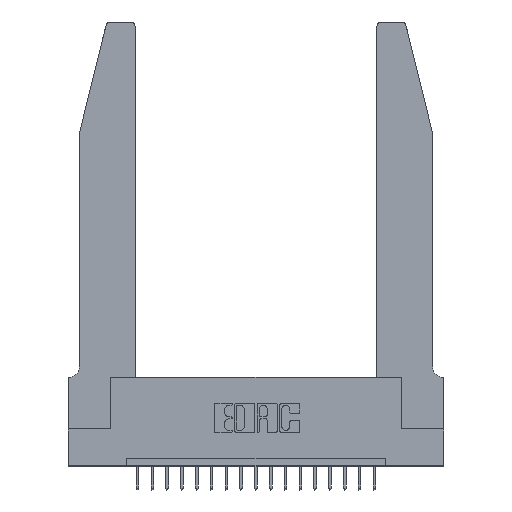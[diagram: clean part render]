
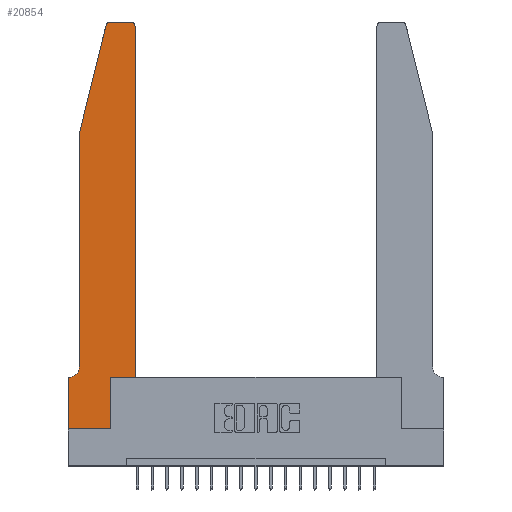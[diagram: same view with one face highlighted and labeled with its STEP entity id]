
A CAD part, top view. The second image highlights one B-rep face of the part: STEP entity #20854.
In plain terms, the highlighted planar face has unit normal (0, 0, 1).
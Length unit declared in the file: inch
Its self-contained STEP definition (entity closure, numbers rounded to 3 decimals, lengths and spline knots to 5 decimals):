
#15 = LINE ( 'NONE', #16925, #7420 ) ;
#464 = DIRECTION ( 'NONE',  ( 0., -1., 0. ) ) ;
#474 = AXIS2_PLACEMENT_3D ( 'NONE', #9435, #6072, #2661 ) ;
#480 = CARTESIAN_POINT ( 'NONE',  ( 0.2865, 0., 0.37 ) ) ;
#1028 = EDGE_CURVE ( 'NONE', #16431, #11741, #10587, .T. ) ;
#1708 = ORIENTED_EDGE ( 'NONE', *, *, #16423, .T. ) ;
#1727 = VERTEX_POINT ( 'NONE', #14026 ) ;
#1805 = CARTESIAN_POINT ( 'NONE',  ( 0.0055, 0.42, 0.37 ) ) ;
#1890 = CARTESIAN_POINT ( 'NONE',  ( 0., 0., 0.37 ) ) ;
#2116 = DIRECTION ( 'NONE',  ( 1., 0., 0. ) ) ;
#2201 = VERTEX_POINT ( 'NONE', #8474 ) ;
#2258 = CARTESIAN_POINT ( 'NONE',  ( 0., 0., 0.37 ) ) ;
#2293 = EDGE_CURVE ( 'NONE', #2201, #3261, #15, .T. ) ;
#2320 = VECTOR ( 'NONE', #464, 39.37008 ) ;
#2518 = FACE_OUTER_BOUND ( 'NONE', #15224, .T. ) ;
#2556 = CARTESIAN_POINT ( 'NONE',  ( 0., 0.35, 0.37 ) ) ;
#2661 = DIRECTION ( 'NONE',  ( 1., 0., 0. ) ) ;
#3010 = EDGE_CURVE ( 'NONE', #5892, #1727, #13741, .T. ) ;
#3032 = LINE ( 'NONE', #14347, #5075 ) ;
#3044 = LINE ( 'NONE', #14842, #20291 ) ;
#3221 = VECTOR ( 'NONE', #3913, 39.37008 ) ;
#3261 = VERTEX_POINT ( 'NONE', #12353 ) ;
#3759 = EDGE_CURVE ( 'NONE', #8178, #20922, #3044, .T. ) ;
#3877 = DIRECTION ( 'NONE',  ( 0., 0., 1. ) ) ;
#3913 = DIRECTION ( 'NONE',  ( -1., 0., 0. ) ) ;
#4110 = ORIENTED_EDGE ( 'NONE', *, *, #18517, .T. ) ;
#4201 = DIRECTION ( 'NONE',  ( 1., 0., 0. ) ) ;
#4340 = CARTESIAN_POINT ( 'NONE',  ( 0.284, 2.75, 0.37 ) ) ;
#5075 = VECTOR ( 'NONE', #9323, 39.37008 ) ;
#5377 = ORIENTED_EDGE ( 'NONE', *, *, #5793, .T. ) ;
#5500 = DIRECTION ( 'NONE',  ( 1., 0., 0. ) ) ;
#5793 = EDGE_CURVE ( 'NONE', #9636, #8731, #16850, .T. ) ;
#5892 = VERTEX_POINT ( 'NONE', #9911 ) ;
#6058 = EDGE_CURVE ( 'NONE', #1727, #16431, #19593, .T. ) ;
#6072 = DIRECTION ( 'NONE',  ( 0., 0., 1. ) ) ;
#6301 = ORIENTED_EDGE ( 'NONE', *, *, #3759, .T. ) ;
#6322 = DIRECTION ( 'NONE',  ( 0., 1., 0. ) ) ;
#6685 = ORIENTED_EDGE ( 'NONE', *, *, #2293, .T. ) ;
#7420 = VECTOR ( 'NONE', #18554, 39.37008 ) ;
#7728 = CARTESIAN_POINT ( 'NONE',  ( 0.0755, 0.35, 0.37 ) ) ;
#7943 = CARTESIAN_POINT ( 'NONE',  ( 0.4505, 2.72, 0.37 ) ) ;
#8092 = EDGE_CURVE ( 'NONE', #8557, #19766, #15757, .T. ) ;
#8126 = AXIS2_PLACEMENT_3D ( 'NONE', #2556, #13939, #4201 ) ;
#8178 = VERTEX_POINT ( 'NONE', #13827 ) ;
#8398 = VECTOR ( 'NONE', #19088, 39.37008 ) ;
#8457 = LINE ( 'NONE', #16055, #17834 ) ;
#8474 = CARTESIAN_POINT ( 'NONE',  ( 0.0755, 2., 0.37 ) ) ;
#8557 = VERTEX_POINT ( 'NONE', #7943 ) ;
#8731 = VERTEX_POINT ( 'NONE', #10074 ) ;
#9323 = DIRECTION ( 'NONE',  ( 0., 1., 0. ) ) ;
#9435 = CARTESIAN_POINT ( 'NONE',  ( 0.284, 2.72, 0.37 ) ) ;
#9636 = VERTEX_POINT ( 'NONE', #4340 ) ;
#9646 = ORIENTED_EDGE ( 'NONE', *, *, #15506, .T. ) ;
#9911 = CARTESIAN_POINT ( 'NONE',  ( 0.0055, 0.35, 0.37 ) ) ;
#10074 = CARTESIAN_POINT ( 'NONE',  ( 0.25487, 2.72718, 0.37 ) ) ;
#10260 = DIRECTION ( 'NONE',  ( 0., 0., -1. ) ) ;
#10293 = AXIS2_PLACEMENT_3D ( 'NONE', #1805, #10260, #10833 ) ;
#10504 = AXIS2_PLACEMENT_3D ( 'NONE', #12119, #3877, #5500 ) ;
#10587 = LINE ( 'NONE', #2258, #10830 ) ;
#10830 = VECTOR ( 'NONE', #2116, 39.37008 ) ;
#10833 = DIRECTION ( 'NONE',  ( -1., 0., 0. ) ) ;
#11424 = ORIENTED_EDGE ( 'NONE', *, *, #1028, .T. ) ;
#11462 = CARTESIAN_POINT ( 'NONE',  ( 0.0755, 2., 0.37 ) ) ;
#11741 = VERTEX_POINT ( 'NONE', #480 ) ;
#11801 = DIRECTION ( 'NONE',  ( 1., 0., 0. ) ) ;
#12119 = CARTESIAN_POINT ( 'NONE',  ( 0.4205, 2.72, 0.37 ) ) ;
#12293 = PLANE ( 'NONE',  #8126 ) ;
#12353 = CARTESIAN_POINT ( 'NONE',  ( 0.0755, 0.42, 0.37 ) ) ;
#12563 = CARTESIAN_POINT ( 'NONE',  ( 0.4505, 0.35, 0.37 ) ) ;
#12831 = ORIENTED_EDGE ( 'NONE', *, *, #3010, .T. ) ;
#12901 = LINE ( 'NONE', #15135, #3221 ) ;
#13422 = CIRCLE ( 'NONE', #10293, 0.07 ) ;
#13741 = LINE ( 'NONE', #7728, #8398 ) ;
#13827 = CARTESIAN_POINT ( 'NONE',  ( 0.2865, 0.35, 0.37 ) ) ;
#13911 = ORIENTED_EDGE ( 'NONE', *, *, #8092, .T. ) ;
#13939 = DIRECTION ( 'NONE',  ( 0., 0., 1. ) ) ;
#14026 = CARTESIAN_POINT ( 'NONE',  ( 0., 0.35, 0.37 ) ) ;
#14347 = CARTESIAN_POINT ( 'NONE',  ( 0.2865, 0.35, 0.37 ) ) ;
#14842 = CARTESIAN_POINT ( 'NONE',  ( 0.4505, 0.35, 0.37 ) ) ;
#15135 = CARTESIAN_POINT ( 'NONE',  ( 0.2605, 2.75, 0.37 ) ) ;
#15224 = EDGE_LOOP ( 'NONE', ( #1708, #5377, #18955, #6685, #9646, #12831, #20210, #11424, #16287, #6301, #4110, #13911 ) ) ;
#15506 = EDGE_CURVE ( 'NONE', #3261, #5892, #13422, .T. ) ;
#15522 = VECTOR ( 'NONE', #17746, 39.37008 ) ;
#15757 = CIRCLE ( 'NONE', #10504, 0.03 ) ;
#16027 = LINE ( 'NONE', #11462, #15522 ) ;
#16055 = CARTESIAN_POINT ( 'NONE',  ( 0.4505, 0.35, 0.37 ) ) ;
#16287 = ORIENTED_EDGE ( 'NONE', *, *, #20892, .T. ) ;
#16421 = CARTESIAN_POINT ( 'NONE',  ( 0.4205, 2.75, 0.37 ) ) ;
#16423 = EDGE_CURVE ( 'NONE', #19766, #9636, #12901, .T. ) ;
#16431 = VERTEX_POINT ( 'NONE', #16772 ) ;
#16772 = CARTESIAN_POINT ( 'NONE',  ( 0., 0., 0.37 ) ) ;
#16850 = CIRCLE ( 'NONE', #474, 0.03 ) ;
#16925 = CARTESIAN_POINT ( 'NONE',  ( 0.0755, 2., 0.37 ) ) ;
#17746 = DIRECTION ( 'NONE',  ( -0.239, -0.971, 0. ) ) ;
#17834 = VECTOR ( 'NONE', #6322, 39.37008 ) ;
#18517 = EDGE_CURVE ( 'NONE', #20922, #8557, #8457, .T. ) ;
#18554 = DIRECTION ( 'NONE',  ( 0., -1., 0. ) ) ;
#18955 = ORIENTED_EDGE ( 'NONE', *, *, #20587, .T. ) ;
#19088 = DIRECTION ( 'NONE',  ( -1., 0., 0. ) ) ;
#19593 = LINE ( 'NONE', #1890, #2320 ) ;
#19766 = VERTEX_POINT ( 'NONE', #16421 ) ;
#20210 = ORIENTED_EDGE ( 'NONE', *, *, #6058, .T. ) ;
#20291 = VECTOR ( 'NONE', #11801, 39.37008 ) ;
#20587 = EDGE_CURVE ( 'NONE', #8731, #2201, #16027, .T. ) ;
#20854 = ADVANCED_FACE ( 'NONE', ( #2518 ), #12293, .T. ) ;
#20892 = EDGE_CURVE ( 'NONE', #11741, #8178, #3032, .T. ) ;
#20922 = VERTEX_POINT ( 'NONE', #12563 ) ;
